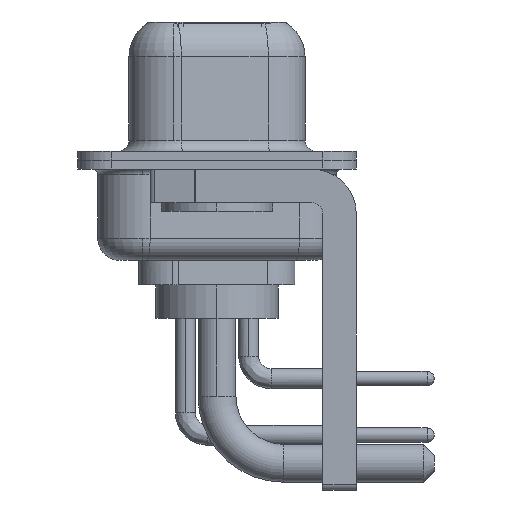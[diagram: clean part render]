
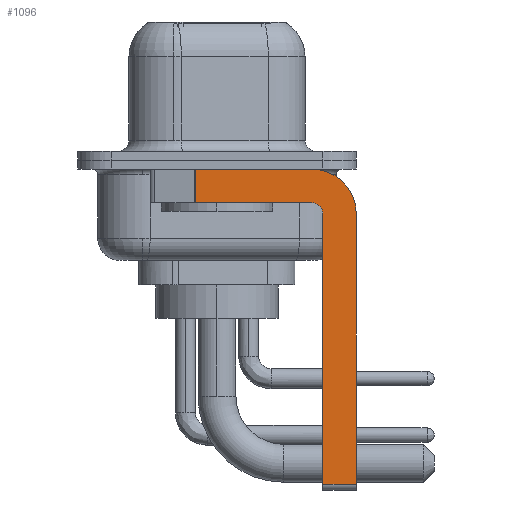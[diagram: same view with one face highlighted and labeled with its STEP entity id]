
A CAD part, left-side view. The second image highlights one B-rep face of the part: STEP entity #1096.
In plain terms, the highlighted planar face has unit normal (-1, 0, 0).
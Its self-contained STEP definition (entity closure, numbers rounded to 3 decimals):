
#146 = VECTOR ( 'NONE', #7837, 1000. ) ;
#552 = VECTOR ( 'NONE', #9935, 1000. ) ;
#711 = VERTEX_POINT ( 'NONE', #20167 ) ;
#917 = ORIENTED_EDGE ( 'NONE', *, *, #5744, .T. ) ;
#1096 = ADVANCED_FACE ( 'NONE', ( #10526 ), #13495, .F. ) ;
#1254 = LINE ( 'NONE', #7805, #19054 ) ;
#1913 = ORIENTED_EDGE ( 'NONE', *, *, #3424, .F. ) ;
#2138 = EDGE_LOOP ( 'NONE', ( #1913, #18664, #17764, #13979, #10141, #917, #3320, #18881 ) ) ;
#2460 = VECTOR ( 'NONE', #14019, 1000. ) ;
#2600 = VERTEX_POINT ( 'NONE', #14312 ) ;
#2819 = CIRCLE ( 'NONE', #16485, 0.5 ) ;
#3193 = DIRECTION ( 'NONE',  ( -1., 0., 0. ) ) ;
#3312 = VERTEX_POINT ( 'NONE', #18381 ) ;
#3320 = ORIENTED_EDGE ( 'NONE', *, *, #15806, .F. ) ;
#3424 = EDGE_CURVE ( 'NONE', #711, #3312, #12169, .T. ) ;
#3442 = CARTESIAN_POINT ( 'NONE',  ( -2.9, -4.25, -2.4 ) ) ;
#3579 = CARTESIAN_POINT ( 'NONE',  ( -2.9, 0.978, -1.9 ) ) ;
#3660 = CARTESIAN_POINT ( 'NONE',  ( -2.9, -4.75, -14.55 ) ) ;
#3929 = CARTESIAN_POINT ( 'NONE',  ( -2.9, 3., -0.4 ) ) ;
#4183 = CARTESIAN_POINT ( 'NONE',  ( -2.9, -6.25, -14.55 ) ) ;
#4464 = LINE ( 'NONE', #9597, #146 ) ;
#4553 = EDGE_CURVE ( 'NONE', #2600, #12910, #2819, .T. ) ;
#4822 = DIRECTION ( 'NONE',  ( 0., -1., 0. ) ) ;
#4832 = DIRECTION ( 'NONE',  ( 0., 0., 1. ) ) ;
#5000 = LINE ( 'NONE', #3579, #552 ) ;
#5149 = CARTESIAN_POINT ( 'NONE',  ( -2.9, -4.75, -14.8 ) ) ;
#5192 = DIRECTION ( 'NONE',  ( 0., 0., -1. ) ) ;
#5744 = EDGE_CURVE ( 'NONE', #15581, #20442, #21570, .T. ) ;
#5797 = EDGE_CURVE ( 'NONE', #15581, #2600, #13384, .T. ) ;
#6564 = CARTESIAN_POINT ( 'NONE',  ( -2.9, -4.25, -14.55 ) ) ;
#7805 = CARTESIAN_POINT ( 'NONE',  ( -2.9, -6.25, -2.4 ) ) ;
#7837 = DIRECTION ( 'NONE',  ( 0., 1., 0. ) ) ;
#7897 = EDGE_CURVE ( 'NONE', #12910, #15641, #4464, .T. ) ;
#8657 = CARTESIAN_POINT ( 'NONE',  ( -2.9, -6.25, -2.4 ) ) ;
#9597 = CARTESIAN_POINT ( 'NONE',  ( -2.9, -4.25, -1.9 ) ) ;
#9935 = DIRECTION ( 'NONE',  ( 0., 0., -1. ) ) ;
#10141 = ORIENTED_EDGE ( 'NONE', *, *, #5797, .F. ) ;
#10526 = FACE_OUTER_BOUND ( 'NONE', #2138, .T. ) ;
#11665 = VERTEX_POINT ( 'NONE', #8657 ) ;
#11966 = DIRECTION ( 'NONE',  ( 0., 0., 1. ) ) ;
#12115 = CIRCLE ( 'NONE', #15600, 2. ) ;
#12169 = LINE ( 'NONE', #3929, #2460 ) ;
#12910 = VERTEX_POINT ( 'NONE', #20909 ) ;
#13283 = CARTESIAN_POINT ( 'NONE',  ( -2.9, -4.25, -2.4 ) ) ;
#13384 = LINE ( 'NONE', #5149, #16482 ) ;
#13495 = PLANE ( 'NONE',  #16718 ) ;
#13979 = ORIENTED_EDGE ( 'NONE', *, *, #4553, .F. ) ;
#14019 = DIRECTION ( 'NONE',  ( 0., -1., 0. ) ) ;
#14312 = CARTESIAN_POINT ( 'NONE',  ( -2.9, -4.75, -2.4 ) ) ;
#14509 = DIRECTION ( 'NONE',  ( 0., 0., -1. ) ) ;
#14618 = CARTESIAN_POINT ( 'NONE',  ( -2.9, 0.978, -1.9 ) ) ;
#14847 = EDGE_CURVE ( 'NONE', #711, #15641, #5000, .T. ) ;
#15454 = VECTOR ( 'NONE', #4822, 1000. ) ;
#15581 = VERTEX_POINT ( 'NONE', #3660 ) ;
#15600 = AXIS2_PLACEMENT_3D ( 'NONE', #3442, #16801, #5192 ) ;
#15641 = VERTEX_POINT ( 'NONE', #14618 ) ;
#15806 = EDGE_CURVE ( 'NONE', #11665, #20442, #1254, .T. ) ;
#16482 = VECTOR ( 'NONE', #11966, 1000. ) ;
#16485 = AXIS2_PLACEMENT_3D ( 'NONE', #13283, #3193, #4832 ) ;
#16718 = AXIS2_PLACEMENT_3D ( 'NONE', #17195, #20357, #16760 ) ;
#16760 = DIRECTION ( 'NONE',  ( 0., 0., -1. ) ) ;
#16801 = DIRECTION ( 'NONE',  ( 1., 0., 0. ) ) ;
#16870 = EDGE_CURVE ( 'NONE', #3312, #11665, #12115, .T. ) ;
#17195 = CARTESIAN_POINT ( 'NONE',  ( -2.9, -4.25, -2.4 ) ) ;
#17764 = ORIENTED_EDGE ( 'NONE', *, *, #7897, .F. ) ;
#18381 = CARTESIAN_POINT ( 'NONE',  ( -2.9, -4.25, -0.4 ) ) ;
#18664 = ORIENTED_EDGE ( 'NONE', *, *, #14847, .T. ) ;
#18881 = ORIENTED_EDGE ( 'NONE', *, *, #16870, .F. ) ;
#19054 = VECTOR ( 'NONE', #14509, 1000. ) ;
#20167 = CARTESIAN_POINT ( 'NONE',  ( -2.9, 0.978, -0.4 ) ) ;
#20357 = DIRECTION ( 'NONE',  ( 1., 0., 0. ) ) ;
#20442 = VERTEX_POINT ( 'NONE', #4183 ) ;
#20909 = CARTESIAN_POINT ( 'NONE',  ( -2.9, -4.25, -1.9 ) ) ;
#21570 = LINE ( 'NONE', #6564, #15454 ) ;
